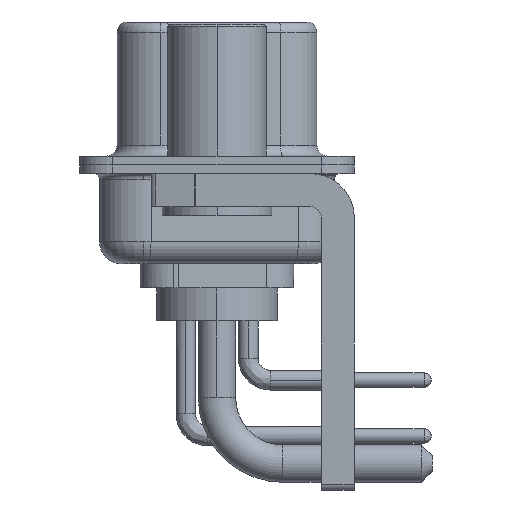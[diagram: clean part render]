
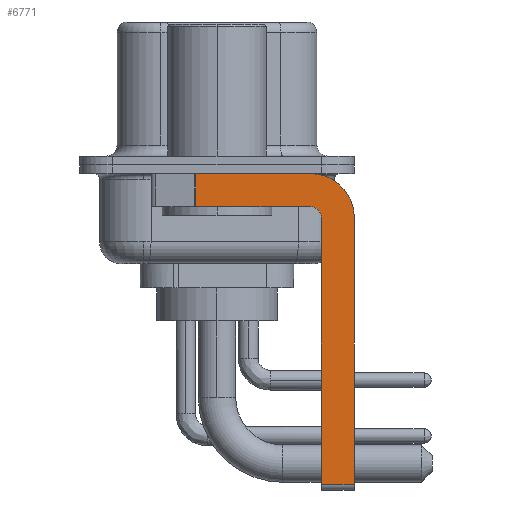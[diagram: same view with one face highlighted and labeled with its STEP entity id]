
A CAD part, left-side view. The second image highlights one B-rep face of the part: STEP entity #6771.
In plain terms, the highlighted planar face has unit normal (-1, 0, 0).
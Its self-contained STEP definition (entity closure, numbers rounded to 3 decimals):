
#143 = CARTESIAN_POINT ( 'NONE',  ( -2.9, 0.978, -1.9 ) ) ;
#175 = CARTESIAN_POINT ( 'NONE',  ( -2.9, 0.978, -0.4 ) ) ;
#286 = EDGE_CURVE ( 'NONE', #27008, #5742, #18880, .T. ) ;
#297 = CARTESIAN_POINT ( 'NONE',  ( -2.9, 0.978, -1.9 ) ) ;
#307 = VECTOR ( 'NONE', #5635, 1000. ) ;
#1457 = VERTEX_POINT ( 'NONE', #25856 ) ;
#1723 = DIRECTION ( 'NONE',  ( 0., -1., 0. ) ) ;
#1778 = CARTESIAN_POINT ( 'NONE',  ( -2.9, -4.75, -2.4 ) ) ;
#2218 = LINE ( 'NONE', #15289, #20578 ) ;
#2880 = ORIENTED_EDGE ( 'NONE', *, *, #15215, .F. ) ;
#3147 = DIRECTION ( 'NONE',  ( 0., 0., -1. ) ) ;
#3275 = VERTEX_POINT ( 'NONE', #1778 ) ;
#4903 = ORIENTED_EDGE ( 'NONE', *, *, #286, .T. ) ;
#5138 = VERTEX_POINT ( 'NONE', #19230 ) ;
#5635 = DIRECTION ( 'NONE',  ( 0., 0., -1. ) ) ;
#5742 = VERTEX_POINT ( 'NONE', #16674 ) ;
#6771 = ADVANCED_FACE ( 'NONE', ( #24094 ), #22036, .F. ) ;
#6968 = CARTESIAN_POINT ( 'NONE',  ( -2.9, -4.25, -2.4 ) ) ;
#7028 = EDGE_CURVE ( 'NONE', #7498, #5742, #16076, .T. ) ;
#7498 = VERTEX_POINT ( 'NONE', #21820 ) ;
#7668 = VECTOR ( 'NONE', #1723, 1000. ) ;
#8408 = DIRECTION ( 'NONE',  ( 0., -1., 0. ) ) ;
#8543 = CARTESIAN_POINT ( 'NONE',  ( -2.9, -4.25, -14.55 ) ) ;
#8763 = CARTESIAN_POINT ( 'NONE',  ( -2.9, -4.25, -2.4 ) ) ;
#8769 = EDGE_LOOP ( 'NONE', ( #2880, #9727, #22408, #12169, #19621, #4903, #17543, #11286 ) ) ;
#8959 = LINE ( 'NONE', #297, #12228 ) ;
#9166 = DIRECTION ( 'NONE',  ( -1., 0., 0. ) ) ;
#9315 = DIRECTION ( 'NONE',  ( 1., 0., 0. ) ) ;
#9439 = EDGE_CURVE ( 'NONE', #5138, #7498, #25678, .T. ) ;
#9727 = ORIENTED_EDGE ( 'NONE', *, *, #24676, .T. ) ;
#11286 = ORIENTED_EDGE ( 'NONE', *, *, #9439, .F. ) ;
#11803 = AXIS2_PLACEMENT_3D ( 'NONE', #6968, #9166, #17559 ) ;
#12169 = ORIENTED_EDGE ( 'NONE', *, *, #21103, .F. ) ;
#12228 = VECTOR ( 'NONE', #21508, 1000. ) ;
#12365 = VERTEX_POINT ( 'NONE', #175 ) ;
#13621 = DIRECTION ( 'NONE',  ( 1., 0., 0. ) ) ;
#15215 = EDGE_CURVE ( 'NONE', #12365, #5138, #24879, .T. ) ;
#15249 = AXIS2_PLACEMENT_3D ( 'NONE', #26181, #13621, #3147 ) ;
#15289 = CARTESIAN_POINT ( 'NONE',  ( -2.9, -4.75, -14.8 ) ) ;
#16076 = LINE ( 'NONE', #24507, #307 ) ;
#16674 = CARTESIAN_POINT ( 'NONE',  ( -2.9, -6.25, -14.55 ) ) ;
#17543 = ORIENTED_EDGE ( 'NONE', *, *, #7028, .F. ) ;
#17559 = DIRECTION ( 'NONE',  ( 0., 0., 1. ) ) ;
#17922 = VECTOR ( 'NONE', #21851, 1000. ) ;
#18880 = LINE ( 'NONE', #8543, #19889 ) ;
#19230 = CARTESIAN_POINT ( 'NONE',  ( -2.9, -4.25, -0.4 ) ) ;
#19621 = ORIENTED_EDGE ( 'NONE', *, *, #24683, .F. ) ;
#19889 = VECTOR ( 'NONE', #8408, 1000. ) ;
#19939 = EDGE_CURVE ( 'NONE', #1457, #22629, #26269, .T. ) ;
#20578 = VECTOR ( 'NONE', #25499, 1000. ) ;
#20599 = CARTESIAN_POINT ( 'NONE',  ( -2.9, 3., -0.4 ) ) ;
#20778 = AXIS2_PLACEMENT_3D ( 'NONE', #8763, #9315, #25583 ) ;
#21103 = EDGE_CURVE ( 'NONE', #3275, #1457, #24581, .T. ) ;
#21508 = DIRECTION ( 'NONE',  ( 0., 0., -1. ) ) ;
#21820 = CARTESIAN_POINT ( 'NONE',  ( -2.9, -6.25, -2.4 ) ) ;
#21851 = DIRECTION ( 'NONE',  ( 0., 1., 0. ) ) ;
#22036 = PLANE ( 'NONE',  #15249 ) ;
#22408 = ORIENTED_EDGE ( 'NONE', *, *, #19939, .F. ) ;
#22629 = VERTEX_POINT ( 'NONE', #143 ) ;
#23905 = CARTESIAN_POINT ( 'NONE',  ( -2.9, -4.25, -1.9 ) ) ;
#24094 = FACE_OUTER_BOUND ( 'NONE', #8769, .T. ) ;
#24507 = CARTESIAN_POINT ( 'NONE',  ( -2.9, -6.25, -2.4 ) ) ;
#24581 = CIRCLE ( 'NONE', #11803, 0.5 ) ;
#24676 = EDGE_CURVE ( 'NONE', #12365, #22629, #8959, .T. ) ;
#24683 = EDGE_CURVE ( 'NONE', #27008, #3275, #2218, .T. ) ;
#24879 = LINE ( 'NONE', #20599, #7668 ) ;
#25499 = DIRECTION ( 'NONE',  ( 0., 0., 1. ) ) ;
#25583 = DIRECTION ( 'NONE',  ( 0., 0., -1. ) ) ;
#25678 = CIRCLE ( 'NONE', #20778, 2. ) ;
#25856 = CARTESIAN_POINT ( 'NONE',  ( -2.9, -4.25, -1.9 ) ) ;
#25859 = CARTESIAN_POINT ( 'NONE',  ( -2.9, -4.75, -14.55 ) ) ;
#26181 = CARTESIAN_POINT ( 'NONE',  ( -2.9, -4.25, -2.4 ) ) ;
#26269 = LINE ( 'NONE', #23905, #17922 ) ;
#27008 = VERTEX_POINT ( 'NONE', #25859 ) ;
